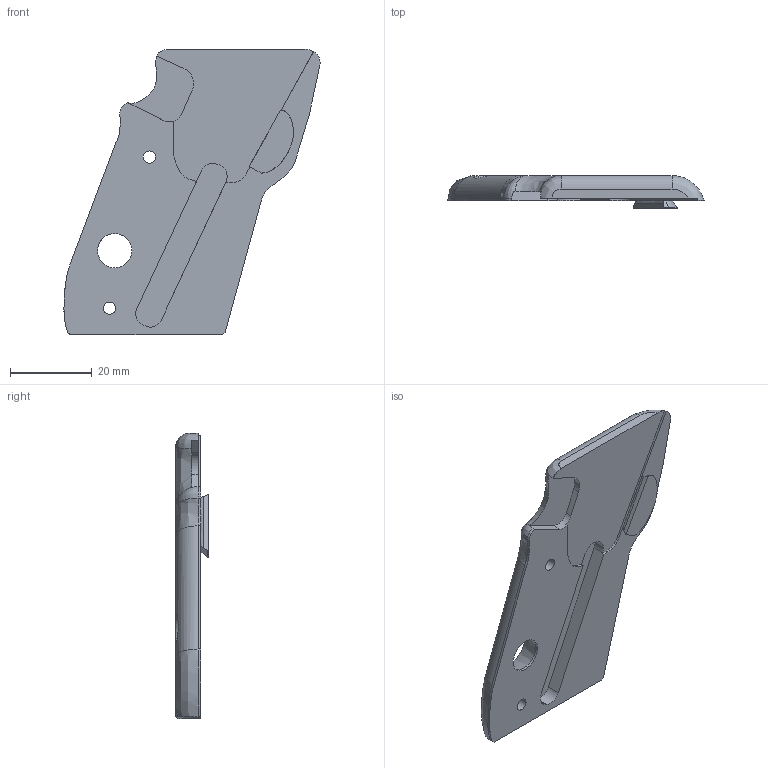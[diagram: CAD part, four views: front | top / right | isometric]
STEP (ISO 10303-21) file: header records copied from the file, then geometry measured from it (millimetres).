
FILE_DESCRIPTION(/* description */ (''),/* implementation_level */ '2;1');
FILE_NAME(/* name */ 'left_grip_final.step',/* time_stamp */ '2021-09-19T17:09:28-04:00',/* author */ (''),/* organization */ (''),/* preprocessor_version */ 'ST-DEVELOPER v18.1',/* originating_system */ 'Autodesk Translation Framework v10.10.0.1391',/* authorisation */ '');
FILE_SCHEMA (('AUTOMOTIVE_DESIGN { 1 0 10303 214 3 1 1 }'));
Length unit declared in the file: millimetre
Products named in the file (1): left_grip
Bounding box: 62.73 x 8 x 69.91 mm (x, y, z)
Volume: 14253.5 mm3; surface area: 7441.2 mm2
Topology: 1 solids, 1 shells, 68 faces, 180 edges, 114 vertices
Faces by surface type: bspline 27, plane 26, cylinder 14, cone 1
Full cylindrical faces by diameter (mm): 3 x2, 6.2 x2, 8.4 x1
Entity records: 3545 total; most frequent: CARTESIAN_POINT 2012, ORIENTED_EDGE 358, DIRECTION 229, EDGE_CURVE 179, VERTEX_POINT 114, LINE 83, VECTOR 83, EDGE_LOOP 75
